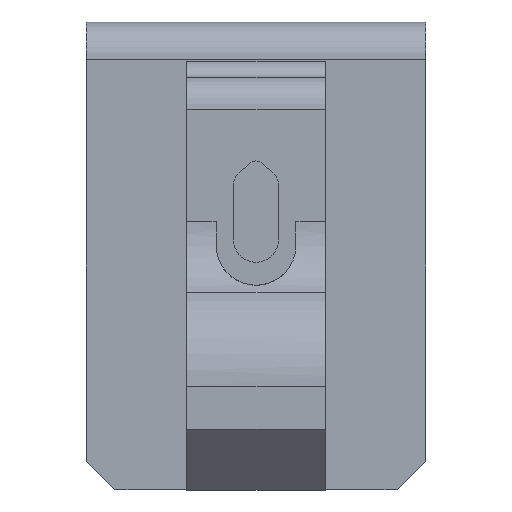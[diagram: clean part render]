
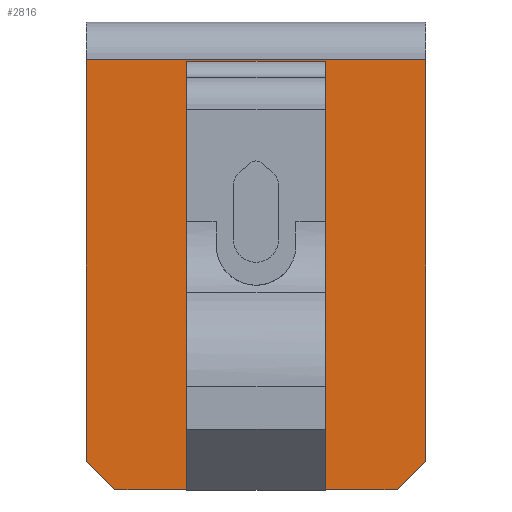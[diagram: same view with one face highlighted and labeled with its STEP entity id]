
A CAD part, front view. The second image highlights one B-rep face of the part: STEP entity #2816.
In plain terms, the highlighted planar face has unit normal (0, -1, 0).
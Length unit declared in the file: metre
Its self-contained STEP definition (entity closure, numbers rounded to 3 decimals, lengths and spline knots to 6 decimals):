
#621=ORIENTED_EDGE('',*,*,#1367,.F.);
#622=ORIENTED_EDGE('',*,*,#1443,.T.);
#623=ORIENTED_EDGE('',*,*,#1374,.F.);
#624=ORIENTED_EDGE('',*,*,#1444,.T.);
#625=ORIENTED_EDGE('',*,*,#1445,.T.);
#626=ORIENTED_EDGE('',*,*,#1409,.F.);
#627=ORIENTED_EDGE('',*,*,#1442,.F.);
#628=ORIENTED_EDGE('',*,*,#1440,.F.);
#629=ORIENTED_EDGE('',*,*,#1446,.T.);
#630=ORIENTED_EDGE('',*,*,#1447,.F.);
#1367=EDGE_CURVE('',#1799,#1800,#2029,.T.);
#1374=EDGE_CURVE('',#1805,#1806,#2033,.T.);
#1409=EDGE_CURVE('',#1828,#1829,#2064,.T.);
#1440=EDGE_CURVE('',#1849,#1850,#2076,.T.);
#1442=EDGE_CURVE('',#1850,#1828,#2077,.T.);
#1443=EDGE_CURVE('',#1799,#1806,#2078,.F.);
#1444=EDGE_CURVE('',#1805,#1851,#2079,.T.);
#1445=EDGE_CURVE('',#1851,#1829,#2080,.F.);
#1446=EDGE_CURVE('',#1849,#1852,#2081,.F.);
#1447=EDGE_CURVE('',#1800,#1852,#2082,.T.);
#1799=VERTEX_POINT('',#4139);
#1800=VERTEX_POINT('',#4141);
#1805=VERTEX_POINT('',#4154);
#1806=VERTEX_POINT('',#4155);
#1828=VERTEX_POINT('',#4228);
#1829=VERTEX_POINT('',#4229);
#1849=VERTEX_POINT('',#4317);
#1850=VERTEX_POINT('',#4319);
#1851=VERTEX_POINT('',#4326);
#1852=VERTEX_POINT('',#4329);
#2029=LINE('',#4140,#2222);
#2033=LINE('',#4153,#2226);
#2064=LINE('',#4227,#2257);
#2076=LINE('',#4318,#2269);
#2077=LINE('',#4322,#2270);
#2078=LINE('',#4324,#2271);
#2079=LINE('',#4325,#2272);
#2080=LINE('',#4327,#2273);
#2081=LINE('',#4328,#2274);
#2082=LINE('',#4330,#2275);
#2222=VECTOR('',#3297,1.);
#2226=VECTOR('',#3309,1.);
#2257=VECTOR('',#3358,1.);
#2269=VECTOR('',#3406,1.);
#2270=VECTOR('',#3411,1.);
#2271=VECTOR('',#3414,1.);
#2272=VECTOR('',#3415,1.);
#2273=VECTOR('',#3416,1.);
#2274=VECTOR('',#3417,1.);
#2275=VECTOR('',#3418,1.);
#2398=EDGE_LOOP('',(#621,#622,#623,#624,#625,#626,#627,#628,#629,#630));
#2576=FACE_BOUND('',#2398,.T.);
#2731=PLANE('',#3036);
#2816=ADVANCED_FACE('',(#2576),#2731,.T.);
#3036=AXIS2_PLACEMENT_3D('',#4323,#3412,#3413);
#3297=DIRECTION('',(0.,0.,-1.));
#3309=DIRECTION('',(0.,0.,1.));
#3358=DIRECTION('',(0.,0.,-1.));
#3406=DIRECTION('',(0.,0.,1.));
#3411=DIRECTION('',(1.,0.,0.));
#3412=DIRECTION('',(0.,-1.,0.));
#3413=DIRECTION('',(0.,0.,-1.));
#3414=DIRECTION('',(-1.,0.,0.));
#3415=DIRECTION('',(1.,0.,0.));
#3416=DIRECTION('',(-0.707,0.,-0.707));
#3417=DIRECTION('',(-0.707,0.,0.707));
#3418=DIRECTION('',(-1.,0.,0.));
#4139=CARTESIAN_POINT('',(-0.015869,0.004729,0.04387));
#4140=CARTESIAN_POINT('',(-0.015869,0.004729,0.025604));
#4141=CARTESIAN_POINT('',(-0.015869,0.004729,0.009821));
#4153=CARTESIAN_POINT('',(-0.004869,0.004729,0.046137));
#4154=CARTESIAN_POINT('',(-0.004869,0.004729,0.009821));
#4155=CARTESIAN_POINT('',(-0.004869,0.004729,0.04387));
#4227=CARTESIAN_POINT('',(0.003131,0.004729,0.050137));
#4228=CARTESIAN_POINT('',(0.003131,0.004729,0.044));
#4229=CARTESIAN_POINT('',(0.003131,0.004729,0.012107));
#4317=CARTESIAN_POINT('',(-0.023869,0.004729,0.012107));
#4318=CARTESIAN_POINT('',(-0.023869,0.004729,0.050137));
#4319=CARTESIAN_POINT('',(-0.023869,0.004729,0.044));
#4322=CARTESIAN_POINT('',(-0.010369,0.004729,0.044));
#4323=CARTESIAN_POINT('',(-0.004869,0.004729,0.050137));
#4324=CARTESIAN_POINT('',(-0.004869,0.004729,0.04387));
#4325=CARTESIAN_POINT('',(0.000131,0.004729,0.009821));
#4326=CARTESIAN_POINT('',(0.000845,0.004729,0.009821));
#4327=CARTESIAN_POINT('',(0.018146,0.004729,0.027122));
#4328=CARTESIAN_POINT('',(-0.033385,0.004729,0.021622));
#4329=CARTESIAN_POINT('',(-0.021583,0.004729,0.009821));
#4330=CARTESIAN_POINT('',(-0.020869,0.004729,0.009821));
